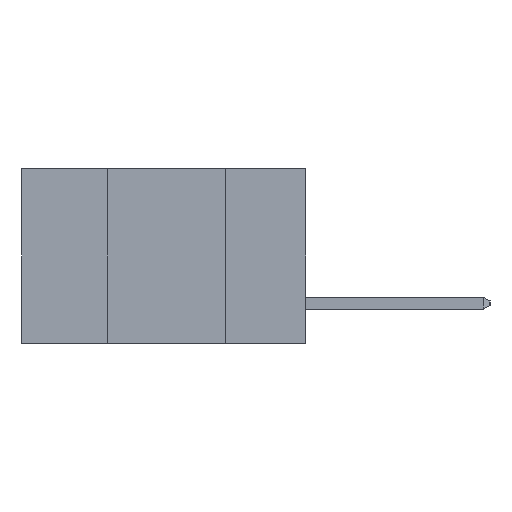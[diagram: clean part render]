
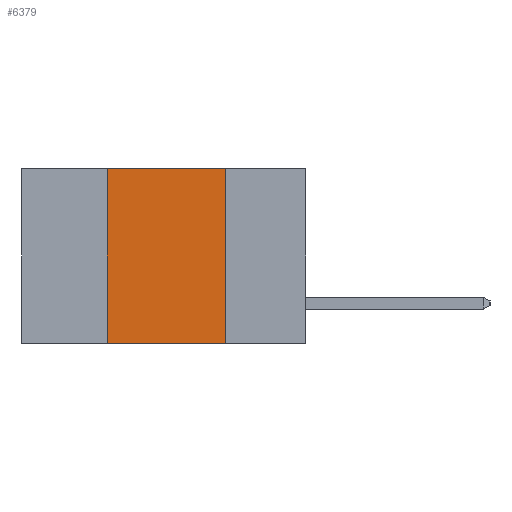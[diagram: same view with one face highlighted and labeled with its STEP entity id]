
A CAD part, left-side view. The second image highlights one B-rep face of the part: STEP entity #6379.
In plain terms, the highlighted planar face has unit normal (-1, 0, 0).
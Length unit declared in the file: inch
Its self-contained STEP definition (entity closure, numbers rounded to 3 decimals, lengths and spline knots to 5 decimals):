
#555 = LINE ( 'NONE', #5304, #3277 ) ;
#580 = FACE_OUTER_BOUND ( 'NONE', #8227, .T. ) ;
#1183 = DIRECTION ( 'NONE',  ( 0., 0., -1. ) ) ;
#1226 = ORIENTED_EDGE ( 'NONE', *, *, #5568, .T. ) ;
#1584 = VECTOR ( 'NONE', #4467, 39.37008 ) ;
#2282 = VERTEX_POINT ( 'NONE', #8616 ) ;
#2702 = CARTESIAN_POINT ( 'NONE',  ( 0., 0.17, -0.37 ) ) ;
#2732 = CARTESIAN_POINT ( 'NONE',  ( 0., 0.17, 0. ) ) ;
#3034 = LINE ( 'NONE', #5454, #5412 ) ;
#3277 = VECTOR ( 'NONE', #7875, 39.37008 ) ;
#3519 = CARTESIAN_POINT ( 'NONE',  ( 0., 0.42, -0.37 ) ) ;
#3633 = ORIENTED_EDGE ( 'NONE', *, *, #7286, .F. ) ;
#3890 = LINE ( 'NONE', #5240, #10515 ) ;
#3927 = PLANE ( 'NONE',  #5105 ) ;
#4051 = LINE ( 'NONE', #3519, #1584 ) ;
#4467 = DIRECTION ( 'NONE',  ( 0., 0., 1. ) ) ;
#4800 = CARTESIAN_POINT ( 'NONE',  ( 0., 0.6, 0. ) ) ;
#5105 = AXIS2_PLACEMENT_3D ( 'NONE', #4800, #6517, #1183 ) ;
#5240 = CARTESIAN_POINT ( 'NONE',  ( 0., 0.6, 0. ) ) ;
#5304 = CARTESIAN_POINT ( 'NONE',  ( 0., 0.17, -0.37 ) ) ;
#5412 = VECTOR ( 'NONE', #10375, 39.37008 ) ;
#5454 = CARTESIAN_POINT ( 'NONE',  ( 0., 0.6, -0.37 ) ) ;
#5525 = VERTEX_POINT ( 'NONE', #2702 ) ;
#5568 = EDGE_CURVE ( 'NONE', #7658, #5525, #3034, .T. ) ;
#5610 = CARTESIAN_POINT ( 'NONE',  ( 0., 0.42, -0.37 ) ) ;
#6136 = EDGE_CURVE ( 'NONE', #7658, #2282, #4051, .T. ) ;
#6379 = ADVANCED_FACE ( 'NONE', ( #580 ), #3927, .F. ) ;
#6517 = DIRECTION ( 'NONE',  ( 1., 0., 0. ) ) ;
#6713 = EDGE_CURVE ( 'NONE', #2282, #10332, #3890, .T. ) ;
#7286 = EDGE_CURVE ( 'NONE', #10332, #5525, #555, .T. ) ;
#7658 = VERTEX_POINT ( 'NONE', #5610 ) ;
#7875 = DIRECTION ( 'NONE',  ( 0., 0., -1. ) ) ;
#8090 = ORIENTED_EDGE ( 'NONE', *, *, #6136, .F. ) ;
#8227 = EDGE_LOOP ( 'NONE', ( #3633, #8978, #8090, #1226 ) ) ;
#8616 = CARTESIAN_POINT ( 'NONE',  ( 0., 0.42, 0. ) ) ;
#8978 = ORIENTED_EDGE ( 'NONE', *, *, #6713, .F. ) ;
#10332 = VERTEX_POINT ( 'NONE', #2732 ) ;
#10375 = DIRECTION ( 'NONE',  ( 0., -1., 0. ) ) ;
#10515 = VECTOR ( 'NONE', #10957, 39.37008 ) ;
#10957 = DIRECTION ( 'NONE',  ( 0., -1., 0. ) ) ;
